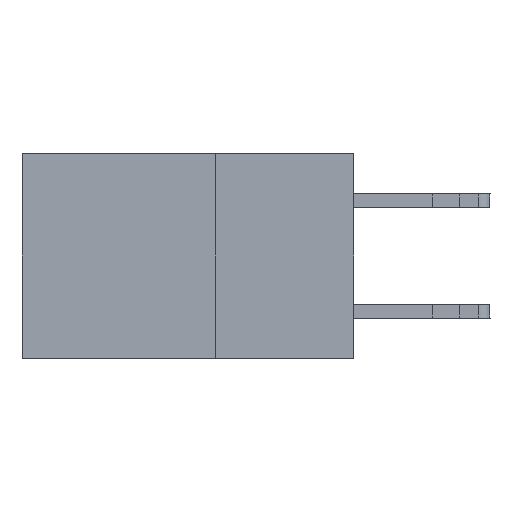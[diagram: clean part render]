
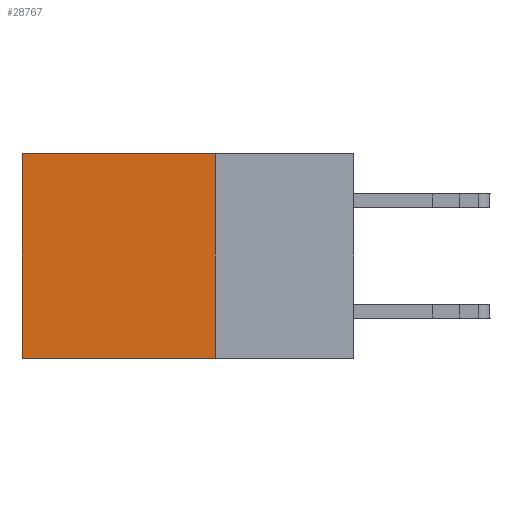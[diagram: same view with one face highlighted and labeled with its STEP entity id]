
A CAD part, left-side view. The second image highlights one B-rep face of the part: STEP entity #28767.
In plain terms, the highlighted planar face has unit normal (-1, 0, 0).
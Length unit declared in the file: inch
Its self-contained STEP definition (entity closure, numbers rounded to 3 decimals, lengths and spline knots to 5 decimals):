
#192 = VERTEX_POINT ( 'NONE', #15766 ) ;
#2894 = PLANE ( 'NONE',  #21871 ) ;
#3488 = CARTESIAN_POINT ( 'NONE',  ( 0.2875, 0.25, 0. ) ) ;
#3918 = VERTEX_POINT ( 'NONE', #13788 ) ;
#4379 = DIRECTION ( 'NONE',  ( 0., 0., -1. ) ) ;
#6673 = VECTOR ( 'NONE', #4379, 39.37008 ) ;
#8134 = EDGE_CURVE ( 'NONE', #31432, #3918, #22625, .T. ) ;
#11059 = ORIENTED_EDGE ( 'NONE', *, *, #8134, .T. ) ;
#12250 = ORIENTED_EDGE ( 'NONE', *, *, #30086, .F. ) ;
#13788 = CARTESIAN_POINT ( 'NONE',  ( 0.2875, 0.6, -0.37 ) ) ;
#15049 = LINE ( 'NONE', #29950, #22877 ) ;
#15766 = CARTESIAN_POINT ( 'NONE',  ( 0.2875, 0.25, -0.37 ) ) ;
#15896 = CARTESIAN_POINT ( 'NONE',  ( 0.2875, 0.6, 0. ) ) ;
#15931 = EDGE_LOOP ( 'NONE', ( #11059, #37332, #12250, #33674 ) ) ;
#16569 = CARTESIAN_POINT ( 'NONE',  ( 0.2875, 0.25, 0. ) ) ;
#17979 = DIRECTION ( 'NONE',  ( 1., 0., 0. ) ) ;
#18762 = FACE_OUTER_BOUND ( 'NONE', #15931, .T. ) ;
#21871 = AXIS2_PLACEMENT_3D ( 'NONE', #3488, #17979, #30479 ) ;
#22250 = EDGE_CURVE ( 'NONE', #27234, #31432, #26138, .T. ) ;
#22625 = LINE ( 'NONE', #15896, #6673 ) ;
#22877 = VECTOR ( 'NONE', #26986, 39.37008 ) ;
#23562 = LINE ( 'NONE', #26556, #33961 ) ;
#26138 = LINE ( 'NONE', #38212, #32574 ) ;
#26556 = CARTESIAN_POINT ( 'NONE',  ( 0.2875, 0.25, 0. ) ) ;
#26986 = DIRECTION ( 'NONE',  ( 0., 1., 0. ) ) ;
#27234 = VERTEX_POINT ( 'NONE', #16569 ) ;
#28767 = ADVANCED_FACE ( 'NONE', ( #18762 ), #2894, .F. ) ;
#29950 = CARTESIAN_POINT ( 'NONE',  ( 0.2875, 0.25, -0.37 ) ) ;
#30086 = EDGE_CURVE ( 'NONE', #27234, #192, #23562, .T. ) ;
#30479 = DIRECTION ( 'NONE',  ( 0., 0., -1. ) ) ;
#31432 = VERTEX_POINT ( 'NONE', #37868 ) ;
#32574 = VECTOR ( 'NONE', #35241, 39.37008 ) ;
#33674 = ORIENTED_EDGE ( 'NONE', *, *, #22250, .T. ) ;
#33961 = VECTOR ( 'NONE', #38630, 39.37008 ) ;
#35241 = DIRECTION ( 'NONE',  ( 0., 1., 0. ) ) ;
#36903 = EDGE_CURVE ( 'NONE', #192, #3918, #15049, .T. ) ;
#37332 = ORIENTED_EDGE ( 'NONE', *, *, #36903, .F. ) ;
#37868 = CARTESIAN_POINT ( 'NONE',  ( 0.2875, 0.6, 0. ) ) ;
#38212 = CARTESIAN_POINT ( 'NONE',  ( 0.2875, 0.25, 0. ) ) ;
#38630 = DIRECTION ( 'NONE',  ( 0., 0., -1. ) ) ;
